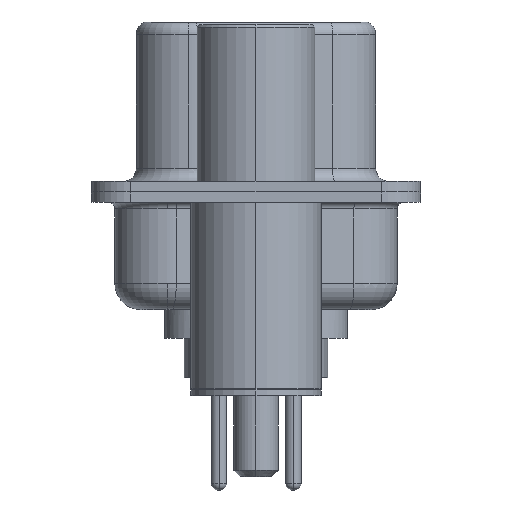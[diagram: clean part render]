
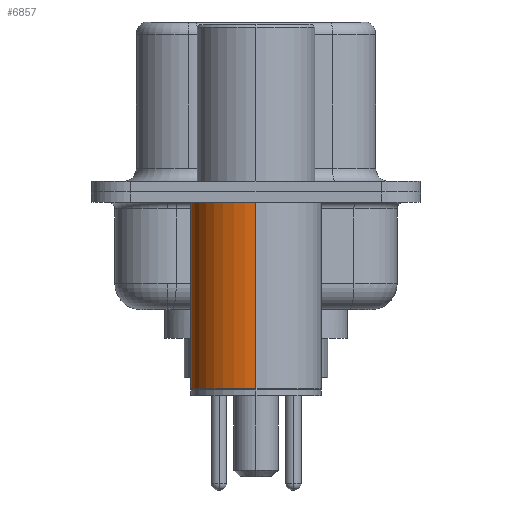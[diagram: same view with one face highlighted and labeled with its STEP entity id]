
A CAD part, left-side view. The second image highlights one B-rep face of the part: STEP entity #6857.
In plain terms, the highlighted cylindrical face has radius 2.5 mm (diameter 5 mm), a partial arc.
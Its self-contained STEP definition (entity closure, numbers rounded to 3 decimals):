
#38 = FACE_OUTER_BOUND ( 'NONE', #847, .T. ) ;
#343 = CIRCLE ( 'NONE', #11023, 2.5 ) ;
#368 = ORIENTED_EDGE ( 'NONE', *, *, #15309, .T. ) ;
#847 = EDGE_LOOP ( 'NONE', ( #5248, #368, #14000, #3979 ) ) ;
#969 = EDGE_CURVE ( 'NONE', #8069, #4821, #343, .T. ) ;
#1667 = DIRECTION ( 'NONE',  ( 0., 0., 1. ) ) ;
#1724 = EDGE_CURVE ( 'NONE', #5033, #8069, #1971, .T. ) ;
#1971 = LINE ( 'NONE', #15188, #11325 ) ;
#1998 = VERTEX_POINT ( 'NONE', #7092 ) ;
#2346 = DIRECTION ( 'NONE',  ( 1., 0., 0. ) ) ;
#3979 = ORIENTED_EDGE ( 'NONE', *, *, #1724, .F. ) ;
#4107 = CARTESIAN_POINT ( 'NONE',  ( 2.5, 0., -0.4 ) ) ;
#4821 = VERTEX_POINT ( 'NONE', #6345 ) ;
#5033 = VERTEX_POINT ( 'NONE', #9545 ) ;
#5248 = ORIENTED_EDGE ( 'NONE', *, *, #15406, .T. ) ;
#6241 = LINE ( 'NONE', #14852, #11485 ) ;
#6345 = CARTESIAN_POINT ( 'NONE',  ( -2.5, 0., -0.4 ) ) ;
#6857 = ADVANCED_FACE ( 'NONE', ( #38 ), #9111, .T. ) ;
#7092 = CARTESIAN_POINT ( 'NONE',  ( -2.5, 0., -7.525 ) ) ;
#7596 = DIRECTION ( 'NONE',  ( 0., 0., 1. ) ) ;
#8069 = VERTEX_POINT ( 'NONE', #4107 ) ;
#8596 = DIRECTION ( 'NONE',  ( 1., 0., 0. ) ) ;
#8971 = CARTESIAN_POINT ( 'NONE',  ( 0., 0., -7.525 ) ) ;
#9111 = CYLINDRICAL_SURFACE ( 'NONE', #13286, 2.5 ) ;
#9545 = CARTESIAN_POINT ( 'NONE',  ( 2.5, 0., -7.525 ) ) ;
#9952 = AXIS2_PLACEMENT_3D ( 'NONE', #8971, #1667, #10199 ) ;
#10199 = DIRECTION ( 'NONE',  ( 1., 0., 0. ) ) ;
#11023 = AXIS2_PLACEMENT_3D ( 'NONE', #15069, #11543, #8596 ) ;
#11325 = VECTOR ( 'NONE', #15223, 1000. ) ;
#11485 = VECTOR ( 'NONE', #7596, 1000. ) ;
#11543 = DIRECTION ( 'NONE',  ( 0., 0., 1. ) ) ;
#13257 = DIRECTION ( 'NONE',  ( 0., 0., 1. ) ) ;
#13286 = AXIS2_PLACEMENT_3D ( 'NONE', #15719, #13257, #2346 ) ;
#13582 = CIRCLE ( 'NONE', #9952, 2.5 ) ;
#14000 = ORIENTED_EDGE ( 'NONE', *, *, #969, .F. ) ;
#14852 = CARTESIAN_POINT ( 'NONE',  ( -2.5, 0., 0.581 ) ) ;
#15069 = CARTESIAN_POINT ( 'NONE',  ( 0., 0., -0.4 ) ) ;
#15188 = CARTESIAN_POINT ( 'NONE',  ( 2.5, 0., 0.581 ) ) ;
#15223 = DIRECTION ( 'NONE',  ( 0., 0., 1. ) ) ;
#15309 = EDGE_CURVE ( 'NONE', #1998, #4821, #6241, .T. ) ;
#15406 = EDGE_CURVE ( 'NONE', #5033, #1998, #13582, .T. ) ;
#15719 = CARTESIAN_POINT ( 'NONE',  ( 0., 0., 0.581 ) ) ;
